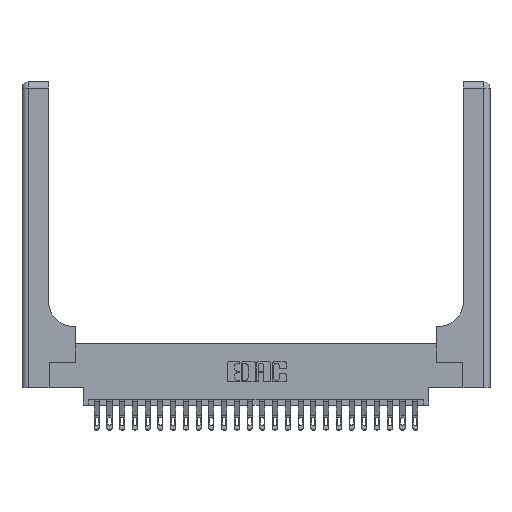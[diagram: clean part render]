
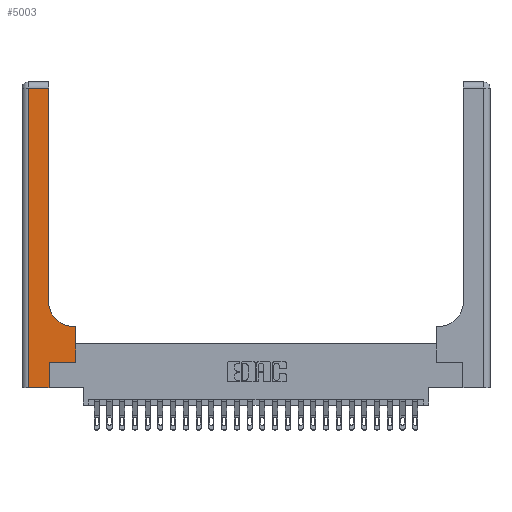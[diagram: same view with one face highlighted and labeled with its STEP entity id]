
A CAD part, top view. The second image highlights one B-rep face of the part: STEP entity #5003.
In plain terms, the highlighted planar face has unit normal (0, 0, 1).
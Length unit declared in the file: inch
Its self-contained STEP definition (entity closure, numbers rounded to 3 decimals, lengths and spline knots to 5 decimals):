
#10 = EDGE_CURVE ( 'NONE', #21762, #14435, #18994, .T. ) ;
#405 = CARTESIAN_POINT ( 'NONE',  ( 0.528, 0.25, 0.37 ) ) ;
#434 = LINE ( 'NONE', #16858, #15281 ) ;
#512 = ORIENTED_EDGE ( 'NONE', *, *, #10, .T. ) ;
#772 = AXIS2_PLACEMENT_3D ( 'NONE', #6951, #20328, #8916 ) ;
#1431 = ORIENTED_EDGE ( 'NONE', *, *, #2763, .T. ) ;
#1597 = CARTESIAN_POINT ( 'NONE',  ( 0., 0., 0.37 ) ) ;
#1713 = DIRECTION ( 'NONE',  ( 0., 1., 0. ) ) ;
#2292 = LINE ( 'NONE', #1597, #8040 ) ;
#2763 = EDGE_CURVE ( 'NONE', #23269, #24418, #4470, .T. ) ;
#3730 = VECTOR ( 'NONE', #8432, 39.37008 ) ;
#4076 = EDGE_CURVE ( 'NONE', #24418, #13224, #2292, .T. ) ;
#4188 = EDGE_CURVE ( 'NONE', #15965, #21447, #4998, .T. ) ;
#4335 = DIRECTION ( 'NONE',  ( 0., 1., 0. ) ) ;
#4470 = LINE ( 'NONE', #7066, #8402 ) ;
#4611 = CARTESIAN_POINT ( 'NONE',  ( 0.528, 0.6, 0.37 ) ) ;
#4998 = LINE ( 'NONE', #405, #19691 ) ;
#5003 = ADVANCED_FACE ( 'NONE', ( #17013 ), #22801, .F. ) ;
#5038 = ORIENTED_EDGE ( 'NONE', *, *, #23991, .T. ) ;
#5223 = DIRECTION ( 'NONE',  ( 0., -1., 0. ) ) ;
#5970 = CARTESIAN_POINT ( 'NONE',  ( 0.26, 2.94, 0.37 ) ) ;
#6430 = EDGE_CURVE ( 'NONE', #12261, #23269, #10115, .T. ) ;
#6469 = CARTESIAN_POINT ( 'NONE',  ( 0., 2.94, 0.37 ) ) ;
#6951 = CARTESIAN_POINT ( 'NONE',  ( 0.51, 0.85, 0.37 ) ) ;
#7031 = ORIENTED_EDGE ( 'NONE', *, *, #6430, .T. ) ;
#7066 = CARTESIAN_POINT ( 'NONE',  ( 0.06, 3., 0.37 ) ) ;
#7252 = DIRECTION ( 'NONE',  ( 0., 1., 0. ) ) ;
#7355 = VECTOR ( 'NONE', #1713, 39.37008 ) ;
#8040 = VECTOR ( 'NONE', #17043, 39.37008 ) ;
#8402 = VECTOR ( 'NONE', #5223, 39.37008 ) ;
#8432 = DIRECTION ( 'NONE',  ( -1., 0., 0. ) ) ;
#8813 = DIRECTION ( 'NONE',  ( 1., 0., 0. ) ) ;
#8916 = DIRECTION ( 'NONE',  ( 1., 0., 0. ) ) ;
#9659 = ORIENTED_EDGE ( 'NONE', *, *, #11314, .T. ) ;
#10115 = LINE ( 'NONE', #6469, #3730 ) ;
#10696 = DIRECTION ( 'NONE',  ( -1., 0., 0. ) ) ;
#10703 = CARTESIAN_POINT ( 'NONE',  ( 0.265, 0.25, 0.37 ) ) ;
#10723 = CARTESIAN_POINT ( 'NONE',  ( 0.26, 0.85, 0.37 ) ) ;
#11314 = EDGE_CURVE ( 'NONE', #23502, #15965, #24355, .T. ) ;
#12203 = CARTESIAN_POINT ( 'NONE',  ( 0.06, 0., 0.37 ) ) ;
#12261 = VERTEX_POINT ( 'NONE', #5970 ) ;
#13224 = VERTEX_POINT ( 'NONE', #24700 ) ;
#13425 = DIRECTION ( 'NONE',  ( -1., 0., 0. ) ) ;
#13432 = CARTESIAN_POINT ( 'NONE',  ( 0.528, 0.25, 0.37 ) ) ;
#13497 = AXIS2_PLACEMENT_3D ( 'NONE', #19027, #24654, #13425 ) ;
#13811 = ORIENTED_EDGE ( 'NONE', *, *, #15749, .T. ) ;
#14435 = VERTEX_POINT ( 'NONE', #10723 ) ;
#14537 = LINE ( 'NONE', #16386, #18944 ) ;
#14948 = EDGE_CURVE ( 'NONE', #21447, #21762, #14537, .T. ) ;
#14962 = EDGE_LOOP ( 'NONE', ( #13811, #7031, #1431, #23013, #5038, #9659, #19031, #15923, #512 ) ) ;
#15281 = VECTOR ( 'NONE', #7252, 39.37008 ) ;
#15749 = EDGE_CURVE ( 'NONE', #14435, #12261, #17617, .T. ) ;
#15923 = ORIENTED_EDGE ( 'NONE', *, *, #14948, .T. ) ;
#15965 = VERTEX_POINT ( 'NONE', #13432 ) ;
#16386 = CARTESIAN_POINT ( 'NONE',  ( 0.26, 0.6, 0.37 ) ) ;
#16858 = CARTESIAN_POINT ( 'NONE',  ( 0.265, 0., 0.37 ) ) ;
#17013 = FACE_OUTER_BOUND ( 'NONE', #14962, .T. ) ;
#17043 = DIRECTION ( 'NONE',  ( 1., 0., 0. ) ) ;
#17617 = LINE ( 'NONE', #22620, #7355 ) ;
#18129 = CARTESIAN_POINT ( 'NONE',  ( 0.06, 2.94, 0.37 ) ) ;
#18944 = VECTOR ( 'NONE', #10696, 39.37008 ) ;
#18994 = CIRCLE ( 'NONE', #772, 0.25 ) ;
#19027 = CARTESIAN_POINT ( 'NONE',  ( 0., 3., 0.37 ) ) ;
#19031 = ORIENTED_EDGE ( 'NONE', *, *, #4188, .T. ) ;
#19393 = VECTOR ( 'NONE', #8813, 39.37008 ) ;
#19691 = VECTOR ( 'NONE', #4335, 39.37008 ) ;
#20328 = DIRECTION ( 'NONE',  ( 0., 0., -1. ) ) ;
#21447 = VERTEX_POINT ( 'NONE', #4611 ) ;
#21762 = VERTEX_POINT ( 'NONE', #22797 ) ;
#22620 = CARTESIAN_POINT ( 'NONE',  ( 0.26, 3., 0.37 ) ) ;
#22797 = CARTESIAN_POINT ( 'NONE',  ( 0.51, 0.6, 0.37 ) ) ;
#22801 = PLANE ( 'NONE',  #13497 ) ;
#22858 = CARTESIAN_POINT ( 'NONE',  ( 0.265, 0.25, 0.37 ) ) ;
#23013 = ORIENTED_EDGE ( 'NONE', *, *, #4076, .T. ) ;
#23269 = VERTEX_POINT ( 'NONE', #18129 ) ;
#23502 = VERTEX_POINT ( 'NONE', #22858 ) ;
#23991 = EDGE_CURVE ( 'NONE', #13224, #23502, #434, .T. ) ;
#24355 = LINE ( 'NONE', #10703, #19393 ) ;
#24418 = VERTEX_POINT ( 'NONE', #12203 ) ;
#24654 = DIRECTION ( 'NONE',  ( 0., 0., -1. ) ) ;
#24700 = CARTESIAN_POINT ( 'NONE',  ( 0.265, 0., 0.37 ) ) ;
